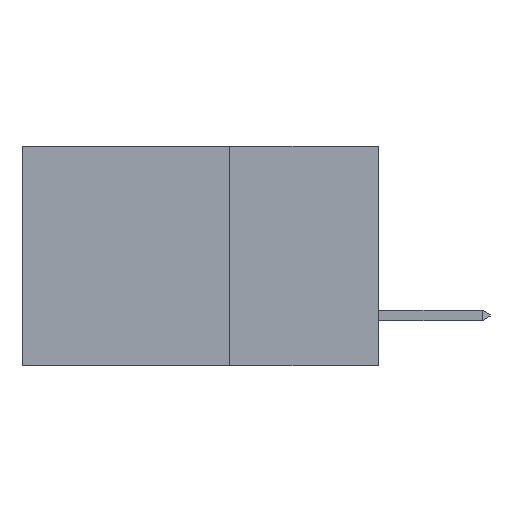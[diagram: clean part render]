
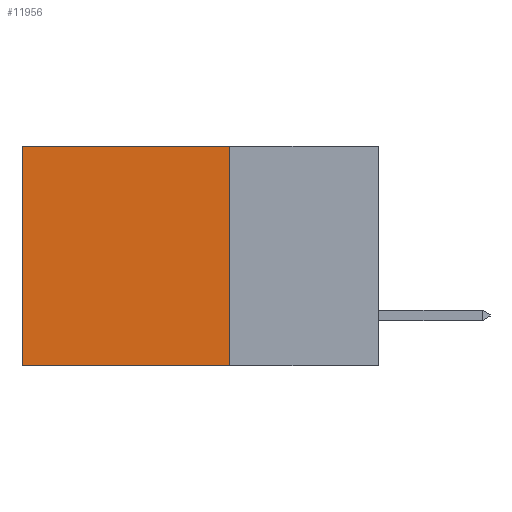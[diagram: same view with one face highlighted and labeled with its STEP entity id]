
A CAD part, left-side view. The second image highlights one B-rep face of the part: STEP entity #11956.
In plain terms, the highlighted planar face has unit normal (-1, 0, 0).
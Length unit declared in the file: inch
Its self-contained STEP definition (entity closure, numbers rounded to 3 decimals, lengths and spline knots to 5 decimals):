
#270 = DIRECTION ( 'NONE',  ( 0., 0., -1. ) ) ;
#342 = CARTESIAN_POINT ( 'NONE',  ( 0.2615, 0.6, 0. ) ) ;
#586 = CARTESIAN_POINT ( 'NONE',  ( 0.2615, 0.25, -0.37 ) ) ;
#588 = ORIENTED_EDGE ( 'NONE', *, *, #3410, .F. ) ;
#1463 = EDGE_CURVE ( 'NONE', #6955, #7005, #5956, .T. ) ;
#1910 = LINE ( 'NONE', #9036, #4308 ) ;
#2098 = VECTOR ( 'NONE', #9779, 39.37008 ) ;
#2243 = EDGE_CURVE ( 'NONE', #8252, #6955, #10246, .T. ) ;
#2307 = PLANE ( 'NONE',  #11489 ) ;
#2328 = ORIENTED_EDGE ( 'NONE', *, *, #2243, .T. ) ;
#2852 = LINE ( 'NONE', #586, #10376 ) ;
#3410 = EDGE_CURVE ( 'NONE', #12385, #7005, #1910, .T. ) ;
#3553 = VECTOR ( 'NONE', #5530, 39.37008 ) ;
#4308 = VECTOR ( 'NONE', #6962, 39.37008 ) ;
#5530 = DIRECTION ( 'NONE',  ( 0., 0., -1. ) ) ;
#5956 = LINE ( 'NONE', #11487, #3553 ) ;
#6406 = DIRECTION ( 'NONE',  ( 1., 0., 0. ) ) ;
#6571 = CARTESIAN_POINT ( 'NONE',  ( 0.2615, 0.6, -0.37 ) ) ;
#6721 = DIRECTION ( 'NONE',  ( 0., 0., -1. ) ) ;
#6955 = VERTEX_POINT ( 'NONE', #342 ) ;
#6962 = DIRECTION ( 'NONE',  ( 0., 1., 0. ) ) ;
#7005 = VERTEX_POINT ( 'NONE', #6571 ) ;
#7146 = CARTESIAN_POINT ( 'NONE',  ( 0.2615, 0.25, 0. ) ) ;
#7483 = FACE_OUTER_BOUND ( 'NONE', #11795, .T. ) ;
#7999 = CARTESIAN_POINT ( 'NONE',  ( 0.2615, 0.25, -0.37 ) ) ;
#8252 = VERTEX_POINT ( 'NONE', #9545 ) ;
#8945 = ORIENTED_EDGE ( 'NONE', *, *, #12160, .F. ) ;
#9036 = CARTESIAN_POINT ( 'NONE',  ( 0.2615, 0.25, -0.37 ) ) ;
#9545 = CARTESIAN_POINT ( 'NONE',  ( 0.2615, 0.25, 0. ) ) ;
#9779 = DIRECTION ( 'NONE',  ( 0., 1., 0. ) ) ;
#10200 = ORIENTED_EDGE ( 'NONE', *, *, #1463, .T. ) ;
#10246 = LINE ( 'NONE', #7146, #2098 ) ;
#10376 = VECTOR ( 'NONE', #6721, 39.37008 ) ;
#11487 = CARTESIAN_POINT ( 'NONE',  ( 0.2615, 0.6, -0.37 ) ) ;
#11489 = AXIS2_PLACEMENT_3D ( 'NONE', #12567, #6406, #270 ) ;
#11795 = EDGE_LOOP ( 'NONE', ( #10200, #588, #8945, #2328 ) ) ;
#11956 = ADVANCED_FACE ( 'NONE', ( #7483 ), #2307, .F. ) ;
#12160 = EDGE_CURVE ( 'NONE', #8252, #12385, #2852, .T. ) ;
#12385 = VERTEX_POINT ( 'NONE', #7999 ) ;
#12567 = CARTESIAN_POINT ( 'NONE',  ( 0.2615, 0.25, -0.37 ) ) ;
